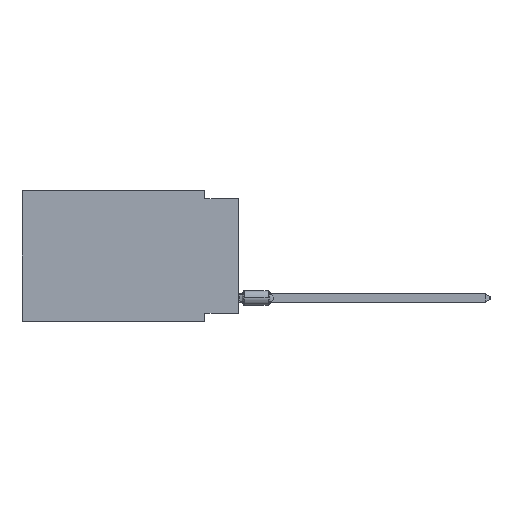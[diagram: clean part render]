
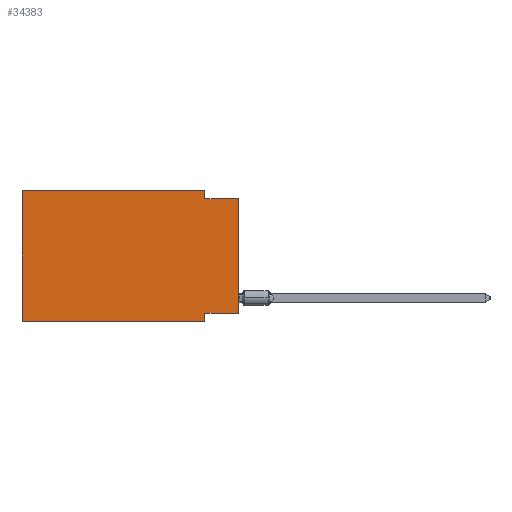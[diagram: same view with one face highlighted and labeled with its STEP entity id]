
A CAD part, left-side view. The second image highlights one B-rep face of the part: STEP entity #34383.
In plain terms, the highlighted planar face has unit normal (-1, 0, 0).
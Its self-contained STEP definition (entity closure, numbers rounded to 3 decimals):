
#1917 = CARTESIAN_POINT ( 'NONE',  ( 0., 16.383, -9.906 ) ) ;
#2817 = EDGE_CURVE ( 'NONE', #30370, #34940, #50081, .T. ) ;
#2973 = AXIS2_PLACEMENT_3D ( 'NONE', #58015, #18315, #24546 ) ;
#3451 = VECTOR ( 'NONE', #33042, 1000. ) ;
#5018 = VERTEX_POINT ( 'NONE', #45555 ) ;
#5977 = ORIENTED_EDGE ( 'NONE', *, *, #2817, .T. ) ;
#6519 = VERTEX_POINT ( 'NONE', #1917 ) ;
#8761 = EDGE_CURVE ( 'NONE', #6519, #43337, #46465, .T. ) ;
#9083 = DIRECTION ( 'NONE',  ( 0., -1., 0. ) ) ;
#9211 = LINE ( 'NONE', #48581, #46683 ) ;
#13185 = VECTOR ( 'NONE', #23191, 1000. ) ;
#13904 = VERTEX_POINT ( 'NONE', #30482 ) ;
#14290 = EDGE_CURVE ( 'NONE', #25617, #14455, #14996, .T. ) ;
#14356 = CARTESIAN_POINT ( 'NONE',  ( 0., 0., 0. ) ) ;
#14455 = VERTEX_POINT ( 'NONE', #23774 ) ;
#14996 = LINE ( 'NONE', #34992, #45388 ) ;
#15517 = VECTOR ( 'NONE', #9083, 1000. ) ;
#15983 = DIRECTION ( 'NONE',  ( 0., -1., 0. ) ) ;
#17599 = LINE ( 'NONE', #37609, #13185 ) ;
#18315 = DIRECTION ( 'NONE',  ( 1., 0., 0. ) ) ;
#21445 = VECTOR ( 'NONE', #15983, 1000. ) ;
#22213 = CARTESIAN_POINT ( 'NONE',  ( 0., 0., -9.271 ) ) ;
#23191 = DIRECTION ( 'NONE',  ( 0., 0., -1. ) ) ;
#23519 = LINE ( 'NONE', #47816, #3451 ) ;
#23774 = CARTESIAN_POINT ( 'NONE',  ( 0., 2.54, -0.635 ) ) ;
#24546 = DIRECTION ( 'NONE',  ( 0., 0., -1. ) ) ;
#24613 = CARTESIAN_POINT ( 'NONE',  ( 0., 0., -0.635 ) ) ;
#24813 = LINE ( 'NONE', #33998, #15517 ) ;
#24868 = EDGE_CURVE ( 'NONE', #6519, #13904, #23519, .T. ) ;
#25617 = VERTEX_POINT ( 'NONE', #53195 ) ;
#28433 = EDGE_LOOP ( 'NONE', ( #5977, #52057, #33139, #40764, #59376, #60940, #58625, #51956 ) ) ;
#30370 = VERTEX_POINT ( 'NONE', #22213 ) ;
#30482 = CARTESIAN_POINT ( 'NONE',  ( 0., 16.383, 0. ) ) ;
#31732 = EDGE_CURVE ( 'NONE', #13904, #25617, #9211, .T. ) ;
#33042 = DIRECTION ( 'NONE',  ( 0., 0., 1. ) ) ;
#33139 = ORIENTED_EDGE ( 'NONE', *, *, #14290, .F. ) ;
#33998 = CARTESIAN_POINT ( 'NONE',  ( 0., 0., -0.635 ) ) ;
#34338 = DIRECTION ( 'NONE',  ( 0., 0., 1. ) ) ;
#34383 = ADVANCED_FACE ( 'NONE', ( #38620 ), #58316, .F. ) ;
#34940 = VERTEX_POINT ( 'NONE', #24613 ) ;
#34992 = CARTESIAN_POINT ( 'NONE',  ( 0., 2.54, 0. ) ) ;
#36153 = CARTESIAN_POINT ( 'NONE',  ( 0., 2.54, -9.906 ) ) ;
#36726 = VECTOR ( 'NONE', #34338, 1000. ) ;
#37609 = CARTESIAN_POINT ( 'NONE',  ( 0., 2.54, -9.906 ) ) ;
#38620 = FACE_OUTER_BOUND ( 'NONE', #28433, .T. ) ;
#40569 = CARTESIAN_POINT ( 'NONE',  ( 0., 16.383, -9.906 ) ) ;
#40764 = ORIENTED_EDGE ( 'NONE', *, *, #31732, .F. ) ;
#43337 = VERTEX_POINT ( 'NONE', #36153 ) ;
#43865 = EDGE_CURVE ( 'NONE', #5018, #43337, #17599, .T. ) ;
#45388 = VECTOR ( 'NONE', #55002, 1000. ) ;
#45555 = CARTESIAN_POINT ( 'NONE',  ( 0., 2.54, -9.271 ) ) ;
#46313 = EDGE_CURVE ( 'NONE', #14455, #34940, #24813, .T. ) ;
#46465 = LINE ( 'NONE', #40569, #21445 ) ;
#46683 = VECTOR ( 'NONE', #54455, 1000. ) ;
#47816 = CARTESIAN_POINT ( 'NONE',  ( 0., 16.383, 0. ) ) ;
#48581 = CARTESIAN_POINT ( 'NONE',  ( 0., 16.383, 0. ) ) ;
#50081 = LINE ( 'NONE', #14356, #36726 ) ;
#51956 = ORIENTED_EDGE ( 'NONE', *, *, #55922, .F. ) ;
#52057 = ORIENTED_EDGE ( 'NONE', *, *, #46313, .F. ) ;
#53195 = CARTESIAN_POINT ( 'NONE',  ( 0., 2.54, 0. ) ) ;
#53333 = DIRECTION ( 'NONE',  ( 0., 1., 0. ) ) ;
#54455 = DIRECTION ( 'NONE',  ( 0., -1., 0. ) ) ;
#55002 = DIRECTION ( 'NONE',  ( 0., 0., -1. ) ) ;
#55922 = EDGE_CURVE ( 'NONE', #30370, #5018, #56962, .T. ) ;
#56123 = VECTOR ( 'NONE', #53333, 1000. ) ;
#56962 = LINE ( 'NONE', #62193, #56123 ) ;
#58015 = CARTESIAN_POINT ( 'NONE',  ( 0., 16.383, 0. ) ) ;
#58316 = PLANE ( 'NONE',  #2973 ) ;
#58625 = ORIENTED_EDGE ( 'NONE', *, *, #43865, .F. ) ;
#59376 = ORIENTED_EDGE ( 'NONE', *, *, #24868, .F. ) ;
#60940 = ORIENTED_EDGE ( 'NONE', *, *, #8761, .T. ) ;
#62193 = CARTESIAN_POINT ( 'NONE',  ( 0., 0., -9.271 ) ) ;
